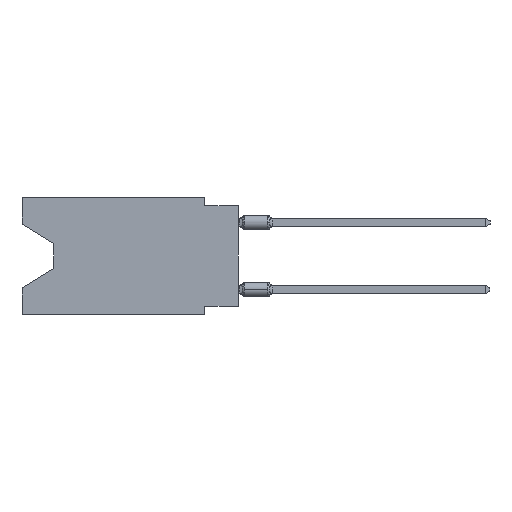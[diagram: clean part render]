
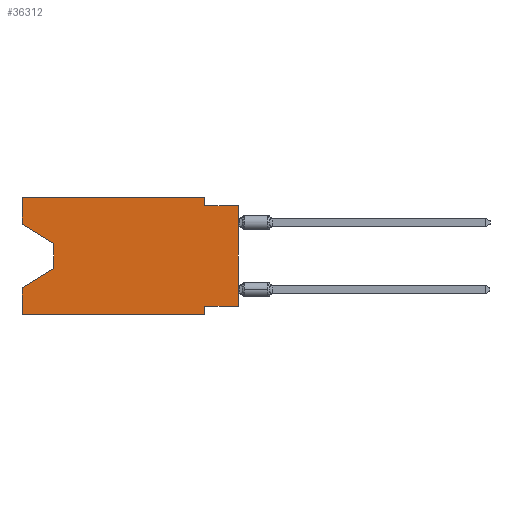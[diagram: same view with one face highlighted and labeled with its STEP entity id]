
A CAD part, left-side view. The second image highlights one B-rep face of the part: STEP entity #36312.
In plain terms, the highlighted planar face has unit normal (-1, 0, 0).
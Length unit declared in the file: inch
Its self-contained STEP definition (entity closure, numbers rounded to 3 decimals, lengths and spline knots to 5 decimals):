
#497 = CARTESIAN_POINT ( 'NONE',  ( 0., 0.1, -0.025 ) ) ;
#894 = DIRECTION ( 'NONE',  ( 0., -1., 0. ) ) ;
#1023 = LINE ( 'NONE', #32933, #48781 ) ;
#4767 = VECTOR ( 'NONE', #56211, 39.37008 ) ;
#5574 = EDGE_CURVE ( 'NONE', #46387, #48548, #15691, .T. ) ;
#5634 = EDGE_CURVE ( 'NONE', #42690, #29660, #22289, .T. ) ;
#6130 = EDGE_CURVE ( 'NONE', #59688, #42690, #1023, .T. ) ;
#8031 = CARTESIAN_POINT ( 'NONE',  ( 0., 0.645, -0.26975 ) ) ;
#8214 = VECTOR ( 'NONE', #30072, 39.37008 ) ;
#8676 = DIRECTION ( 'NONE',  ( 0., 0.855, -0.519 ) ) ;
#9026 = CARTESIAN_POINT ( 'NONE',  ( 0., 0.645, 0. ) ) ;
#9502 = VERTEX_POINT ( 'NONE', #18104 ) ;
#9699 = EDGE_CURVE ( 'NONE', #54605, #54153, #25614, .T. ) ;
#10095 = DIRECTION ( 'NONE',  ( 0., 0., 1. ) ) ;
#11118 = VECTOR ( 'NONE', #36546, 39.37008 ) ;
#13020 = ORIENTED_EDGE ( 'NONE', *, *, #32652, .F. ) ;
#14078 = ORIENTED_EDGE ( 'NONE', *, *, #6130, .T. ) ;
#14444 = VERTEX_POINT ( 'NONE', #55852 ) ;
#15248 = VERTEX_POINT ( 'NONE', #35976 ) ;
#15691 = LINE ( 'NONE', #28683, #50865 ) ;
#17614 = VECTOR ( 'NONE', #33279, 39.37008 ) ;
#18056 = VECTOR ( 'NONE', #10095, 39.37008 ) ;
#18104 = CARTESIAN_POINT ( 'NONE',  ( 0., 0.645, 0. ) ) ;
#19964 = LINE ( 'NONE', #34217, #18056 ) ;
#20345 = ORIENTED_EDGE ( 'NONE', *, *, #9699, .T. ) ;
#21766 = EDGE_CURVE ( 'NONE', #9502, #15248, #27864, .T. ) ;
#21943 = AXIS2_PLACEMENT_3D ( 'NONE', #28496, #51963, #28781 ) ;
#22289 = LINE ( 'NONE', #50996, #34091 ) ;
#22795 = EDGE_CURVE ( 'NONE', #14444, #54153, #33960, .T. ) ;
#25572 = LINE ( 'NONE', #52776, #33244 ) ;
#25614 = LINE ( 'NONE', #49396, #34148 ) ;
#25744 = CARTESIAN_POINT ( 'NONE',  ( 0., 0., 0. ) ) ;
#26721 = ORIENTED_EDGE ( 'NONE', *, *, #22795, .F. ) ;
#27355 = VECTOR ( 'NONE', #42451, 39.37008 ) ;
#27864 = LINE ( 'NONE', #9026, #11118 ) ;
#28496 = CARTESIAN_POINT ( 'NONE',  ( 0., 0.645, 0. ) ) ;
#28683 = CARTESIAN_POINT ( 'NONE',  ( 0., 0., -0.025 ) ) ;
#28781 = DIRECTION ( 'NONE',  ( 0., 0., -1. ) ) ;
#29660 = VERTEX_POINT ( 'NONE', #8031 ) ;
#30072 = DIRECTION ( 'NONE',  ( 0., 0., 1. ) ) ;
#30619 = EDGE_CURVE ( 'NONE', #15248, #46387, #25572, .T. ) ;
#30677 = ORIENTED_EDGE ( 'NONE', *, *, #5634, .T. ) ;
#30689 = LINE ( 'NONE', #25744, #8214 ) ;
#30855 = DIRECTION ( 'NONE',  ( 0., -1., 0. ) ) ;
#31221 = EDGE_CURVE ( 'NONE', #42244, #9502, #42150, .T. ) ;
#31296 = ORIENTED_EDGE ( 'NONE', *, *, #52358, .F. ) ;
#32652 = EDGE_CURVE ( 'NONE', #38797, #14444, #38210, .T. ) ;
#32933 = CARTESIAN_POINT ( 'NONE',  ( 0., 0.55, -0.138 ) ) ;
#33123 = ORIENTED_EDGE ( 'NONE', *, *, #5574, .F. ) ;
#33244 = VECTOR ( 'NONE', #33641, 39.37008 ) ;
#33279 = DIRECTION ( 'NONE',  ( 0., 1., 0. ) ) ;
#33641 = DIRECTION ( 'NONE',  ( 0., 0., -1. ) ) ;
#33790 = ORIENTED_EDGE ( 'NONE', *, *, #31221, .F. ) ;
#33960 = LINE ( 'NONE', #42602, #4767 ) ;
#34091 = VECTOR ( 'NONE', #8676, 39.37008 ) ;
#34148 = VECTOR ( 'NONE', #30855, 39.37008 ) ;
#34217 = CARTESIAN_POINT ( 'NONE',  ( 0., 0.645, 0. ) ) ;
#35976 = CARTESIAN_POINT ( 'NONE',  ( 0., 0.1, 0. ) ) ;
#36312 = ADVANCED_FACE ( 'NONE', ( #37748 ), #36824, .F. ) ;
#36546 = DIRECTION ( 'NONE',  ( 0., -1., 0. ) ) ;
#36796 = ORIENTED_EDGE ( 'NONE', *, *, #21766, .F. ) ;
#36824 = PLANE ( 'NONE',  #21943 ) ;
#37182 = CARTESIAN_POINT ( 'NONE',  ( 0., 0.1, -0.35 ) ) ;
#37356 = EDGE_CURVE ( 'NONE', #38797, #48548, #30689, .T. ) ;
#37748 = FACE_OUTER_BOUND ( 'NONE', #43528, .T. ) ;
#38202 = ORIENTED_EDGE ( 'NONE', *, *, #37356, .T. ) ;
#38210 = LINE ( 'NONE', #43144, #17614 ) ;
#38797 = VERTEX_POINT ( 'NONE', #60014 ) ;
#39593 = VECTOR ( 'NONE', #58733, 39.37008 ) ;
#42150 = LINE ( 'NONE', #50483, #27355 ) ;
#42244 = VERTEX_POINT ( 'NONE', #59721 ) ;
#42451 = DIRECTION ( 'NONE',  ( 0., 0., 1. ) ) ;
#42548 = EDGE_CURVE ( 'NONE', #42244, #59688, #44520, .T. ) ;
#42602 = CARTESIAN_POINT ( 'NONE',  ( 0., 0.1, -0.35 ) ) ;
#42690 = VERTEX_POINT ( 'NONE', #50373 ) ;
#43144 = CARTESIAN_POINT ( 'NONE',  ( 0., 0., -0.325 ) ) ;
#43528 = EDGE_LOOP ( 'NONE', ( #53976, #14078, #30677, #31296, #20345, #26721, #13020, #38202, #33123, #53223, #36796, #33790 ) ) ;
#44520 = LINE ( 'NONE', #44833, #39593 ) ;
#44833 = CARTESIAN_POINT ( 'NONE',  ( 0., 0.645, -0.08025 ) ) ;
#45767 = CARTESIAN_POINT ( 'NONE',  ( 0., 0.645, -0.35 ) ) ;
#46387 = VERTEX_POINT ( 'NONE', #497 ) ;
#46832 = DIRECTION ( 'NONE',  ( 0., 0., -1. ) ) ;
#48548 = VERTEX_POINT ( 'NONE', #54638 ) ;
#48781 = VECTOR ( 'NONE', #46832, 39.37008 ) ;
#49396 = CARTESIAN_POINT ( 'NONE',  ( 0., 0.645, -0.35 ) ) ;
#50373 = CARTESIAN_POINT ( 'NONE',  ( 0., 0.55, -0.212 ) ) ;
#50483 = CARTESIAN_POINT ( 'NONE',  ( 0., 0.645, 0. ) ) ;
#50865 = VECTOR ( 'NONE', #894, 39.37008 ) ;
#50996 = CARTESIAN_POINT ( 'NONE',  ( 0., 0.55, -0.212 ) ) ;
#51963 = DIRECTION ( 'NONE',  ( 1., 0., 0. ) ) ;
#52358 = EDGE_CURVE ( 'NONE', #54605, #29660, #19964, .T. ) ;
#52776 = CARTESIAN_POINT ( 'NONE',  ( 0., 0.1, 0. ) ) ;
#53223 = ORIENTED_EDGE ( 'NONE', *, *, #30619, .F. ) ;
#53976 = ORIENTED_EDGE ( 'NONE', *, *, #42548, .T. ) ;
#54153 = VERTEX_POINT ( 'NONE', #37182 ) ;
#54605 = VERTEX_POINT ( 'NONE', #45767 ) ;
#54638 = CARTESIAN_POINT ( 'NONE',  ( 0., 0., -0.025 ) ) ;
#55852 = CARTESIAN_POINT ( 'NONE',  ( 0., 0.1, -0.325 ) ) ;
#56211 = DIRECTION ( 'NONE',  ( 0., 0., -1. ) ) ;
#58733 = DIRECTION ( 'NONE',  ( 0., -0.855, -0.519 ) ) ;
#59551 = CARTESIAN_POINT ( 'NONE',  ( 0., 0.55, -0.138 ) ) ;
#59688 = VERTEX_POINT ( 'NONE', #59551 ) ;
#59721 = CARTESIAN_POINT ( 'NONE',  ( 0., 0.645, -0.08025 ) ) ;
#60014 = CARTESIAN_POINT ( 'NONE',  ( 0., 0., -0.325 ) ) ;
